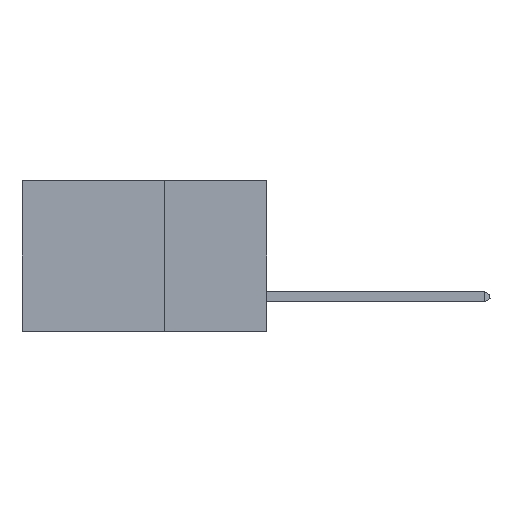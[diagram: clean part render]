
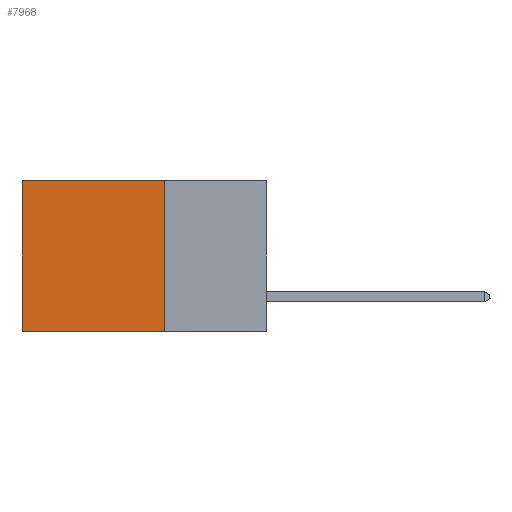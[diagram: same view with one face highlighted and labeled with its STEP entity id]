
A CAD part, left-side view. The second image highlights one B-rep face of the part: STEP entity #7968.
In plain terms, the highlighted planar face has unit normal (-1, 0, 0).
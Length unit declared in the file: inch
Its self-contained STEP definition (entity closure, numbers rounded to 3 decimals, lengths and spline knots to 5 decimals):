
#923 = CARTESIAN_POINT ( 'NONE',  ( 0.2875, 0.25, 0. ) ) ;
#1176 = CARTESIAN_POINT ( 'NONE',  ( 0.2875, 0.6, 0. ) ) ;
#2669 = PLANE ( 'NONE',  #13998 ) ;
#2737 = CARTESIAN_POINT ( 'NONE',  ( 0.2875, 0.6, -0.37 ) ) ;
#2928 = ORIENTED_EDGE ( 'NONE', *, *, #4910, .T. ) ;
#4910 = EDGE_CURVE ( 'NONE', #12441, #16374, #18612, .T. ) ;
#5537 = DIRECTION ( 'NONE',  ( 0., 1., 0. ) ) ;
#7764 = VECTOR ( 'NONE', #9339, 39.37008 ) ;
#7968 = ADVANCED_FACE ( 'NONE', ( #20949 ), #2669, .F. ) ;
#8130 = DIRECTION ( 'NONE',  ( 0., 0., -1. ) ) ;
#8232 = CARTESIAN_POINT ( 'NONE',  ( 0.2875, 0.25, -0.37 ) ) ;
#8338 = VECTOR ( 'NONE', #5537, 39.37008 ) ;
#8489 = CARTESIAN_POINT ( 'NONE',  ( 0.2875, 0.25, 0. ) ) ;
#8637 = CARTESIAN_POINT ( 'NONE',  ( 0.2875, 0.25, 0. ) ) ;
#9339 = DIRECTION ( 'NONE',  ( 0., 0., -1. ) ) ;
#9861 = ORIENTED_EDGE ( 'NONE', *, *, #19558, .T. ) ;
#10264 = DIRECTION ( 'NONE',  ( 0., 0., -1. ) ) ;
#10333 = VECTOR ( 'NONE', #10264, 39.37008 ) ;
#10789 = VERTEX_POINT ( 'NONE', #2737 ) ;
#11157 = ORIENTED_EDGE ( 'NONE', *, *, #18128, .F. ) ;
#11336 = EDGE_LOOP ( 'NONE', ( #9861, #16461, #11157, #2928 ) ) ;
#12441 = VERTEX_POINT ( 'NONE', #21038 ) ;
#12706 = CARTESIAN_POINT ( 'NONE',  ( 0.2875, 0.25, -0.37 ) ) ;
#13998 = AXIS2_PLACEMENT_3D ( 'NONE', #923, #18922, #8130 ) ;
#14457 = EDGE_CURVE ( 'NONE', #17175, #10789, #16124, .T. ) ;
#14511 = LINE ( 'NONE', #8489, #10333 ) ;
#16124 = LINE ( 'NONE', #12706, #8338 ) ;
#16374 = VERTEX_POINT ( 'NONE', #1176 ) ;
#16461 = ORIENTED_EDGE ( 'NONE', *, *, #14457, .F. ) ;
#17175 = VERTEX_POINT ( 'NONE', #8232 ) ;
#17513 = VECTOR ( 'NONE', #22892, 39.37008 ) ;
#17799 = LINE ( 'NONE', #21962, #7764 ) ;
#18128 = EDGE_CURVE ( 'NONE', #12441, #17175, #14511, .T. ) ;
#18612 = LINE ( 'NONE', #8637, #17513 ) ;
#18922 = DIRECTION ( 'NONE',  ( 1., 0., 0. ) ) ;
#19558 = EDGE_CURVE ( 'NONE', #16374, #10789, #17799, .T. ) ;
#20949 = FACE_OUTER_BOUND ( 'NONE', #11336, .T. ) ;
#21038 = CARTESIAN_POINT ( 'NONE',  ( 0.2875, 0.25, 0. ) ) ;
#21962 = CARTESIAN_POINT ( 'NONE',  ( 0.2875, 0.6, 0. ) ) ;
#22892 = DIRECTION ( 'NONE',  ( 0., 1., 0. ) ) ;
